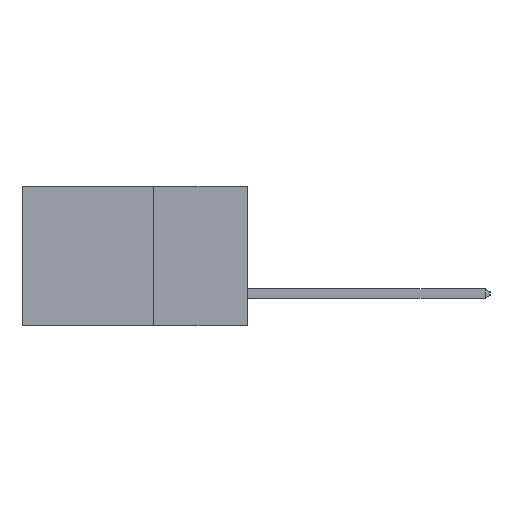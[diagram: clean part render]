
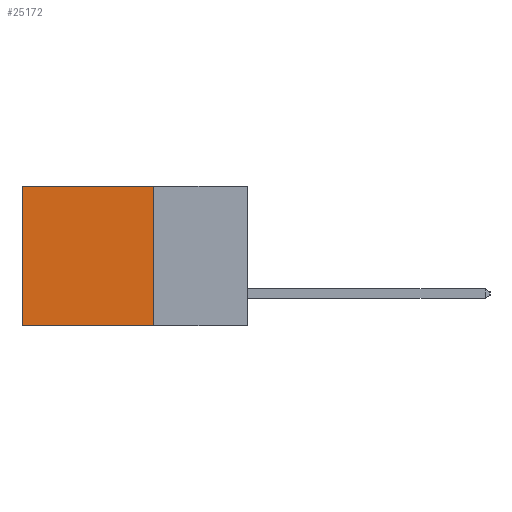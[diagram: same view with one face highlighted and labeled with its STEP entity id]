
A CAD part, left-side view. The second image highlights one B-rep face of the part: STEP entity #25172.
In plain terms, the highlighted planar face has unit normal (-1, 0, 0).
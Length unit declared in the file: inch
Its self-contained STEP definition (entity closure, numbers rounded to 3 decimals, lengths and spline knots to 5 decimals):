
#500 = PLANE ( 'NONE',  #20676 ) ;
#1486 = ORIENTED_EDGE ( 'NONE', *, *, #25090, .T. ) ;
#1527 = LINE ( 'NONE', #17874, #13030 ) ;
#4748 = DIRECTION ( 'NONE',  ( 0., 0., -1. ) ) ;
#6689 = CARTESIAN_POINT ( 'NONE',  ( 0.298, 0.25, 0. ) ) ;
#6752 = EDGE_CURVE ( 'NONE', #19917, #15044, #1527, .T. ) ;
#6784 = VECTOR ( 'NONE', #22889, 39.37008 ) ;
#8035 = LINE ( 'NONE', #18947, #6784 ) ;
#10107 = EDGE_CURVE ( 'NONE', #15692, #15044, #18555, .T. ) ;
#13030 = VECTOR ( 'NONE', #19855, 39.37008 ) ;
#14595 = CARTESIAN_POINT ( 'NONE',  ( 0.298, 0.25, 0. ) ) ;
#14849 = VECTOR ( 'NONE', #16644, 39.37008 ) ;
#15044 = VERTEX_POINT ( 'NONE', #19172 ) ;
#15579 = VERTEX_POINT ( 'NONE', #19153 ) ;
#15692 = VERTEX_POINT ( 'NONE', #23544 ) ;
#16171 = EDGE_CURVE ( 'NONE', #15579, #19917, #8035, .T. ) ;
#16644 = DIRECTION ( 'NONE',  ( 0., 1., 0. ) ) ;
#16915 = DIRECTION ( 'NONE',  ( 1., 0., 0. ) ) ;
#17874 = CARTESIAN_POINT ( 'NONE',  ( 0.298, 0.25, -0.37 ) ) ;
#17948 = VECTOR ( 'NONE', #21384, 39.37008 ) ;
#18337 = FACE_OUTER_BOUND ( 'NONE', #20243, .T. ) ;
#18555 = LINE ( 'NONE', #25362, #17948 ) ;
#18947 = CARTESIAN_POINT ( 'NONE',  ( 0.298, 0.25, 0. ) ) ;
#19153 = CARTESIAN_POINT ( 'NONE',  ( 0.298, 0.25, 0. ) ) ;
#19172 = CARTESIAN_POINT ( 'NONE',  ( 0.298, 0.6, -0.37 ) ) ;
#19855 = DIRECTION ( 'NONE',  ( 0., 1., 0. ) ) ;
#19917 = VERTEX_POINT ( 'NONE', #23772 ) ;
#20243 = EDGE_LOOP ( 'NONE', ( #25366, #24413, #20835, #1486 ) ) ;
#20676 = AXIS2_PLACEMENT_3D ( 'NONE', #6689, #16915, #4748 ) ;
#20835 = ORIENTED_EDGE ( 'NONE', *, *, #16171, .F. ) ;
#21384 = DIRECTION ( 'NONE',  ( 0., 0., -1. ) ) ;
#22889 = DIRECTION ( 'NONE',  ( 0., 0., -1. ) ) ;
#23544 = CARTESIAN_POINT ( 'NONE',  ( 0.298, 0.6, 0. ) ) ;
#23772 = CARTESIAN_POINT ( 'NONE',  ( 0.298, 0.25, -0.37 ) ) ;
#24413 = ORIENTED_EDGE ( 'NONE', *, *, #6752, .F. ) ;
#25090 = EDGE_CURVE ( 'NONE', #15579, #15692, #25570, .T. ) ;
#25172 = ADVANCED_FACE ( 'NONE', ( #18337 ), #500, .F. ) ;
#25362 = CARTESIAN_POINT ( 'NONE',  ( 0.298, 0.6, 0. ) ) ;
#25366 = ORIENTED_EDGE ( 'NONE', *, *, #10107, .T. ) ;
#25570 = LINE ( 'NONE', #14595, #14849 ) ;
